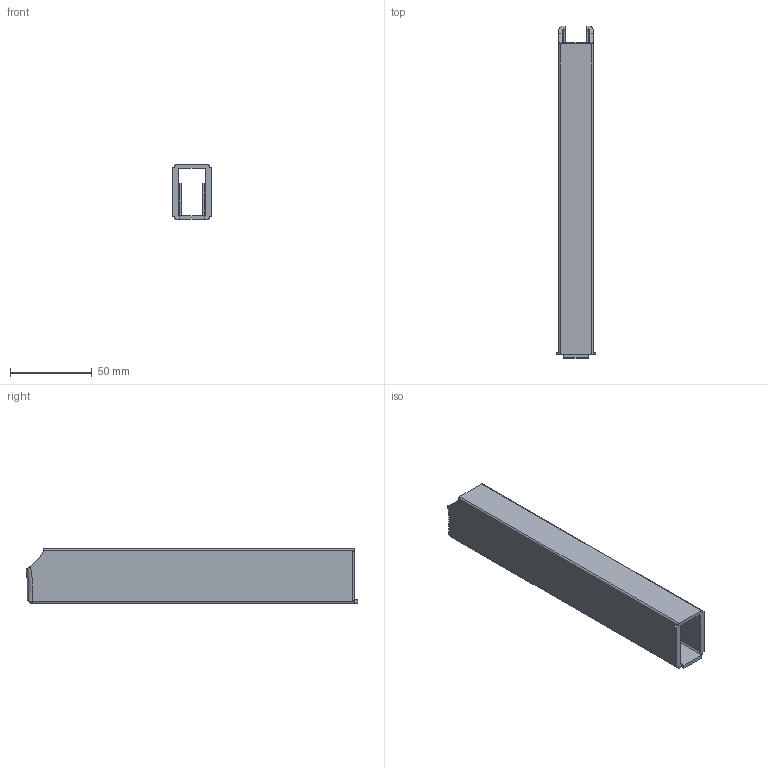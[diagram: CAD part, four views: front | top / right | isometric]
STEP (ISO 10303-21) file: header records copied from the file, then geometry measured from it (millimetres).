
FILE_DESCRIPTION (( 'STEP AP214' ), '1' );
FILE_NAME ('mag_body_AR.STEP', '2013-06-03T01:10:19', ( '' ), ( '' ), 'SwSTEP 2.0', 'SolidWorks 2013', '' );
FILE_SCHEMA (( 'AUTOMOTIVE_DESIGN' ));
Length unit declared in the file: millimetre
Products named in the file (1): mag_body_AR
Bounding box: 24 x 202.81 x 33.5 mm (x, y, z)
Volume: 40987.2 mm3; surface area: 39403.1 mm2
Topology: 1 solids, 1 shells, 207 faces, 576 edges, 376 vertices
Faces by surface type: plane 95, bspline 79, cylinder 29, sphere 2, torus 2
Entity records: 11610 total; most frequent: CARTESIAN_POINT 6809, ORIENTED_EDGE 1140, DIRECTION 716, EDGE_CURVE 570, VERTEX_POINT 374, LINE 350, VECTOR 350, EDGE_LOOP 230
